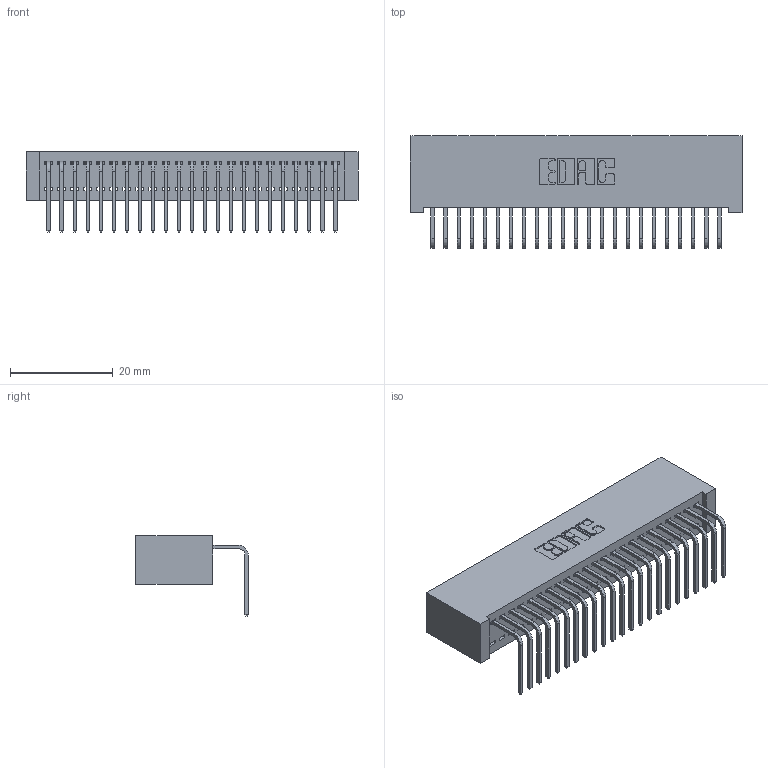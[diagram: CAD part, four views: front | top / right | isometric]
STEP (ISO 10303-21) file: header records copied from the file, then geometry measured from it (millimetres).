
FILE_DESCRIPTION (( 'STEP AP203' ), '1' );
FILE_NAME ('392-023-558-101.STEP', '2019-10-07T06:59:45', ( '' ), ( '' ), 'SwSTEP 2.0', 'SolidWorks 2016', '' );
FILE_SCHEMA (( 'CONFIG_CONTROL_DESIGN' ));
Length unit declared in the file: inch
Products named in the file (3): 392-023-558-101; 342 Part_Lugless; 345-292-001_558 Tail - 2
Assembly tree (24 placements, depth 2):
  392-023-558-101
    342 Part_Lugless
    345-292-001_558 Tail - 2  x23
Bounding box: 64.67 x 21.91 x 15.62 mm (x, y, z)
Volume: 6085.7 mm3; surface area: 9340.4 mm2
Topology: 24 solids, 24 shells, 1482 faces, 4461 edges, 2942 vertices
Faces by surface type: plane 1074, cylinder 408
Entity records: 16193 total; most frequent: CARTESIAN_POINT 2803, ORIENTED_EDGE 2762, DIRECTION 2395, EDGE_CURVE 1381, VECTOR 1261, LINE 1261, VERTEX_POINT 918, AXIS2_PLACEMENT_3D 567
